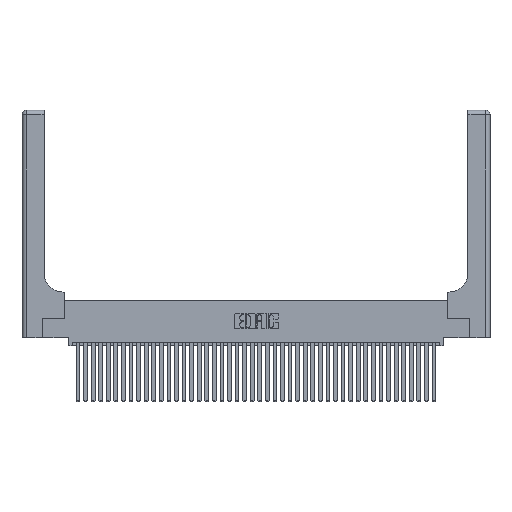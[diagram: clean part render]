
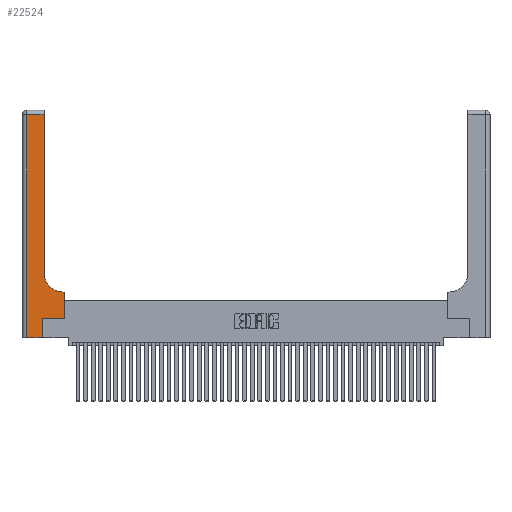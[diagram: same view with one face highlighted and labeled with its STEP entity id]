
A CAD part, top view. The second image highlights one B-rep face of the part: STEP entity #22524.
In plain terms, the highlighted planar face has unit normal (0, 0, 1).
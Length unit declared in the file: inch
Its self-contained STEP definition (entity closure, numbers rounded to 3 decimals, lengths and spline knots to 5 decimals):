
#57 = CARTESIAN_POINT ( 'NONE',  ( 0.269, 0., 0.37 ) ) ;
#1614 = CARTESIAN_POINT ( 'NONE',  ( 0.2915, 3., 0.37 ) ) ;
#2469 = LINE ( 'NONE', #17217, #35979 ) ;
#3299 = DIRECTION ( 'NONE',  ( 0., 0., -1. ) ) ;
#3495 = CARTESIAN_POINT ( 'NONE',  ( 0.5415, 0.6, 0.37 ) ) ;
#3600 = VECTOR ( 'NONE', #32549, 39.37008 ) ;
#5282 = CARTESIAN_POINT ( 'NONE',  ( 0., 0., 0.37 ) ) ;
#7241 = CARTESIAN_POINT ( 'NONE',  ( 0.269, 0.25, 0.37 ) ) ;
#7552 = DIRECTION ( 'NONE',  ( -1., 0., 0. ) ) ;
#7666 = VERTEX_POINT ( 'NONE', #26750 ) ;
#8164 = VECTOR ( 'NONE', #34604, 39.37008 ) ;
#9628 = EDGE_LOOP ( 'NONE', ( #20362, #13378, #24481, #33205, #40880, #16440, #32836, #34814, #30523 ) ) ;
#11218 = LINE ( 'NONE', #14399, #30610 ) ;
#11323 = DIRECTION ( 'NONE',  ( 0., 1., 0. ) ) ;
#11787 = EDGE_CURVE ( 'NONE', #13684, #40308, #25714, .T. ) ;
#11911 = EDGE_CURVE ( 'NONE', #7666, #35519, #13969, .T. ) ;
#12144 = LINE ( 'NONE', #57, #3600 ) ;
#12465 = VERTEX_POINT ( 'NONE', #34912 ) ;
#13378 = ORIENTED_EDGE ( 'NONE', *, *, #32116, .T. ) ;
#13684 = VERTEX_POINT ( 'NONE', #31994 ) ;
#13969 = LINE ( 'NONE', #15596, #21624 ) ;
#14399 = CARTESIAN_POINT ( 'NONE',  ( 0.5585, 0.25, 0.37 ) ) ;
#14952 = AXIS2_PLACEMENT_3D ( 'NONE', #22712, #3299, #26003 ) ;
#14995 = CARTESIAN_POINT ( 'NONE',  ( 0., 3., 0.37 ) ) ;
#15042 = DIRECTION ( 'NONE',  ( 1., 0., 0. ) ) ;
#15263 = AXIS2_PLACEMENT_3D ( 'NONE', #14995, #37752, #18251 ) ;
#15406 = CARTESIAN_POINT ( 'NONE',  ( 0.2915, 0.85, 0.37 ) ) ;
#15596 = CARTESIAN_POINT ( 'NONE',  ( 0.2915, 0.6, 0.37 ) ) ;
#15871 = CARTESIAN_POINT ( 'NONE',  ( 0.2915, 2.94, 0.37 ) ) ;
#16440 = ORIENTED_EDGE ( 'NONE', *, *, #37635, .T. ) ;
#16802 = FACE_OUTER_BOUND ( 'NONE', #9628, .T. ) ;
#17044 = VECTOR ( 'NONE', #15042, 39.37008 ) ;
#17217 = CARTESIAN_POINT ( 'NONE',  ( 0., 2.94, 0.37 ) ) ;
#18251 = DIRECTION ( 'NONE',  ( -1., 0., 0. ) ) ;
#18559 = CIRCLE ( 'NONE', #14952, 0.25 ) ;
#20362 = ORIENTED_EDGE ( 'NONE', *, *, #40471, .T. ) ;
#21624 = VECTOR ( 'NONE', #38364, 39.37008 ) ;
#21823 = VECTOR ( 'NONE', #26782, 39.37008 ) ;
#22524 = ADVANCED_FACE ( 'NONE', ( #16802 ), #31234, .F. ) ;
#22564 = EDGE_CURVE ( 'NONE', #12465, #13684, #33112, .T. ) ;
#22712 = CARTESIAN_POINT ( 'NONE',  ( 0.5415, 0.85, 0.37 ) ) ;
#24481 = ORIENTED_EDGE ( 'NONE', *, *, #22564, .T. ) ;
#24794 = CARTESIAN_POINT ( 'NONE',  ( 0.5585, 0.25, 0.37 ) ) ;
#25714 = LINE ( 'NONE', #5282, #17044 ) ;
#26003 = DIRECTION ( 'NONE',  ( 1., 0., 0. ) ) ;
#26750 = CARTESIAN_POINT ( 'NONE',  ( 0.5585, 0.6, 0.37 ) ) ;
#26782 = DIRECTION ( 'NONE',  ( 1., 0., 0. ) ) ;
#28183 = VERTEX_POINT ( 'NONE', #15871 ) ;
#28719 = VERTEX_POINT ( 'NONE', #15406 ) ;
#29047 = EDGE_CURVE ( 'NONE', #29657, #7666, #11218, .T. ) ;
#29657 = VERTEX_POINT ( 'NONE', #24794 ) ;
#30432 = VECTOR ( 'NONE', #11323, 39.37008 ) ;
#30478 = LINE ( 'NONE', #7241, #21823 ) ;
#30523 = ORIENTED_EDGE ( 'NONE', *, *, #33484, .T. ) ;
#30610 = VECTOR ( 'NONE', #37153, 39.37008 ) ;
#30665 = EDGE_CURVE ( 'NONE', #40308, #30685, #12144, .T. ) ;
#30685 = VERTEX_POINT ( 'NONE', #39207 ) ;
#31234 = PLANE ( 'NONE',  #15263 ) ;
#31382 = CARTESIAN_POINT ( 'NONE',  ( 0.06, 3., 0.37 ) ) ;
#31994 = CARTESIAN_POINT ( 'NONE',  ( 0.06, 0., 0.37 ) ) ;
#32116 = EDGE_CURVE ( 'NONE', #28183, #12465, #2469, .T. ) ;
#32549 = DIRECTION ( 'NONE',  ( 0., 1., 0. ) ) ;
#32836 = ORIENTED_EDGE ( 'NONE', *, *, #29047, .T. ) ;
#33112 = LINE ( 'NONE', #31382, #8164 ) ;
#33136 = CARTESIAN_POINT ( 'NONE',  ( 0.269, 0., 0.37 ) ) ;
#33205 = ORIENTED_EDGE ( 'NONE', *, *, #11787, .T. ) ;
#33484 = EDGE_CURVE ( 'NONE', #35519, #28719, #18559, .T. ) ;
#34604 = DIRECTION ( 'NONE',  ( 0., -1., 0. ) ) ;
#34814 = ORIENTED_EDGE ( 'NONE', *, *, #11911, .T. ) ;
#34912 = CARTESIAN_POINT ( 'NONE',  ( 0.06, 2.94, 0.37 ) ) ;
#35519 = VERTEX_POINT ( 'NONE', #3495 ) ;
#35979 = VECTOR ( 'NONE', #7552, 39.37008 ) ;
#37153 = DIRECTION ( 'NONE',  ( 0., 1., 0. ) ) ;
#37635 = EDGE_CURVE ( 'NONE', #30685, #29657, #30478, .T. ) ;
#37752 = DIRECTION ( 'NONE',  ( 0., 0., -1. ) ) ;
#38364 = DIRECTION ( 'NONE',  ( -1., 0., 0. ) ) ;
#39059 = LINE ( 'NONE', #1614, #30432 ) ;
#39207 = CARTESIAN_POINT ( 'NONE',  ( 0.269, 0.25, 0.37 ) ) ;
#40308 = VERTEX_POINT ( 'NONE', #33136 ) ;
#40471 = EDGE_CURVE ( 'NONE', #28719, #28183, #39059, .T. ) ;
#40880 = ORIENTED_EDGE ( 'NONE', *, *, #30665, .T. ) ;
